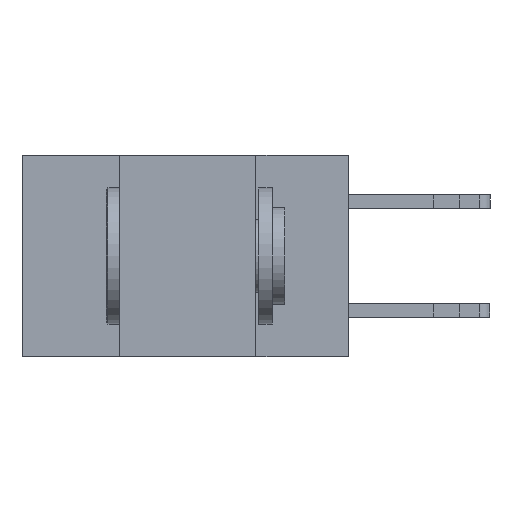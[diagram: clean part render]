
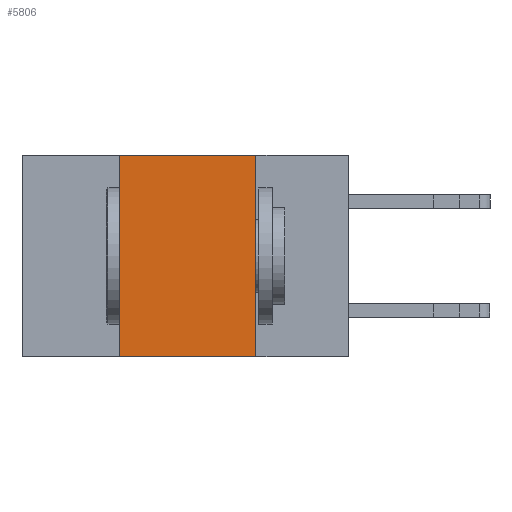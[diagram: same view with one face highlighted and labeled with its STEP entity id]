
A CAD part, left-side view. The second image highlights one B-rep face of the part: STEP entity #5806.
In plain terms, the highlighted planar face has unit normal (-1, 0, 0).
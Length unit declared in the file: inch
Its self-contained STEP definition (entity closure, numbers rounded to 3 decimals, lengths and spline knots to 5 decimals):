
#176 = CARTESIAN_POINT ( 'NONE',  ( 0., 0.17, 0. ) ) ;
#288 = VERTEX_POINT ( 'NONE', #12148 ) ;
#522 = VECTOR ( 'NONE', #8741, 39.37008 ) ;
#748 = ORIENTED_EDGE ( 'NONE', *, *, #11314, .T. ) ;
#851 = VECTOR ( 'NONE', #9503, 39.37008 ) ;
#1204 = CARTESIAN_POINT ( 'NONE',  ( 0., 0.6, -0.37 ) ) ;
#1206 = ORIENTED_EDGE ( 'NONE', *, *, #11381, .F. ) ;
#1311 = DIRECTION ( 'NONE',  ( 0., 0., 1. ) ) ;
#2486 = VECTOR ( 'NONE', #1311, 39.37008 ) ;
#3055 = LINE ( 'NONE', #176, #8399 ) ;
#3135 = CARTESIAN_POINT ( 'NONE',  ( 0., 0.6, 0. ) ) ;
#3214 = ORIENTED_EDGE ( 'NONE', *, *, #10664, .F. ) ;
#3515 = EDGE_LOOP ( 'NONE', ( #3214, #4724, #1206, #748 ) ) ;
#3593 = DIRECTION ( 'NONE',  ( 1., 0., 0. ) ) ;
#3781 = DIRECTION ( 'NONE',  ( 0., 0., -1. ) ) ;
#4724 = ORIENTED_EDGE ( 'NONE', *, *, #12476, .F. ) ;
#4843 = VERTEX_POINT ( 'NONE', #11942 ) ;
#5136 = AXIS2_PLACEMENT_3D ( 'NONE', #7339, #3593, #3781 ) ;
#5374 = LINE ( 'NONE', #6748, #2486 ) ;
#5806 = ADVANCED_FACE ( 'NONE', ( #13133 ), #8021, .F. ) ;
#6355 = LINE ( 'NONE', #1204, #522 ) ;
#6748 = CARTESIAN_POINT ( 'NONE',  ( 0., 0.42, 0. ) ) ;
#7339 = CARTESIAN_POINT ( 'NONE',  ( 0., 0.6, 0. ) ) ;
#7832 = LINE ( 'NONE', #3135, #851 ) ;
#8021 = PLANE ( 'NONE',  #5136 ) ;
#8399 = VECTOR ( 'NONE', #8851, 39.37008 ) ;
#8741 = DIRECTION ( 'NONE',  ( 0., -1., 0. ) ) ;
#8851 = DIRECTION ( 'NONE',  ( 0., 0., -1. ) ) ;
#9503 = DIRECTION ( 'NONE',  ( 0., -1., 0. ) ) ;
#10049 = CARTESIAN_POINT ( 'NONE',  ( 0., 0.42, -0.37 ) ) ;
#10325 = VERTEX_POINT ( 'NONE', #11493 ) ;
#10664 = EDGE_CURVE ( 'NONE', #288, #10325, #3055, .T. ) ;
#11314 = EDGE_CURVE ( 'NONE', #13680, #10325, #6355, .T. ) ;
#11381 = EDGE_CURVE ( 'NONE', #13680, #4843, #5374, .T. ) ;
#11493 = CARTESIAN_POINT ( 'NONE',  ( 0., 0.17, -0.37 ) ) ;
#11942 = CARTESIAN_POINT ( 'NONE',  ( 0., 0.42, 0. ) ) ;
#12148 = CARTESIAN_POINT ( 'NONE',  ( 0., 0.17, 0. ) ) ;
#12476 = EDGE_CURVE ( 'NONE', #4843, #288, #7832, .T. ) ;
#13133 = FACE_OUTER_BOUND ( 'NONE', #3515, .T. ) ;
#13680 = VERTEX_POINT ( 'NONE', #10049 ) ;
